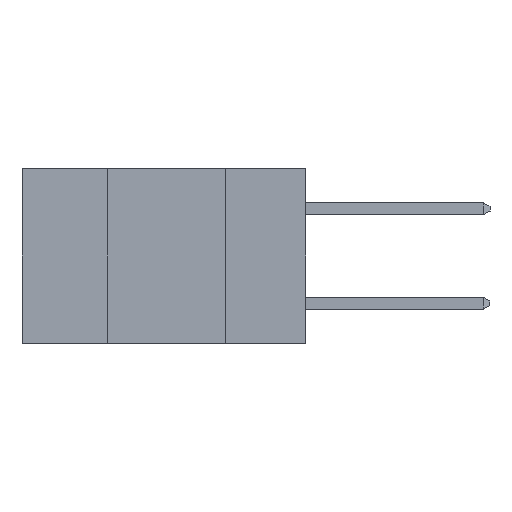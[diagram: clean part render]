
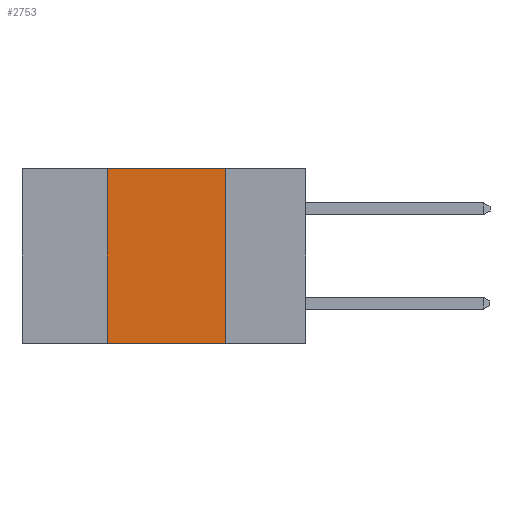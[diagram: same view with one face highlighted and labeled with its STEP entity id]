
A CAD part, left-side view. The second image highlights one B-rep face of the part: STEP entity #2753.
In plain terms, the highlighted planar face has unit normal (-1, 0, 0).
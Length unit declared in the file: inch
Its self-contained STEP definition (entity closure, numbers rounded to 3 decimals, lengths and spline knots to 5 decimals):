
#71 = VECTOR ( 'NONE', #6612, 39.37008 ) ;
#269 = VECTOR ( 'NONE', #9009, 39.37008 ) ;
#537 = CARTESIAN_POINT ( 'NONE',  ( 0., 0.6, -0.37 ) ) ;
#635 = VECTOR ( 'NONE', #5246, 39.37008 ) ;
#1013 = ORIENTED_EDGE ( 'NONE', *, *, #5475, .F. ) ;
#1156 = DIRECTION ( 'NONE',  ( 1., 0., 0. ) ) ;
#1180 = LINE ( 'NONE', #12051, #8700 ) ;
#1385 = PLANE ( 'NONE',  #6379 ) ;
#2689 = EDGE_LOOP ( 'NONE', ( #1013, #3523, #4507, #5567 ) ) ;
#2753 = ADVANCED_FACE ( 'NONE', ( #4590 ), #1385, .F. ) ;
#3091 = CARTESIAN_POINT ( 'NONE',  ( 0., 0.42, 0. ) ) ;
#3523 = ORIENTED_EDGE ( 'NONE', *, *, #11080, .F. ) ;
#3814 = DIRECTION ( 'NONE',  ( 0., 0., -1. ) ) ;
#4144 = VERTEX_POINT ( 'NONE', #3091 ) ;
#4183 = EDGE_CURVE ( 'NONE', #7644, #7170, #6390, .T. ) ;
#4507 = ORIENTED_EDGE ( 'NONE', *, *, #4842, .F. ) ;
#4590 = FACE_OUTER_BOUND ( 'NONE', #2689, .T. ) ;
#4842 = EDGE_CURVE ( 'NONE', #7644, #4144, #1180, .T. ) ;
#5246 = DIRECTION ( 'NONE',  ( 0., -1., 0. ) ) ;
#5475 = EDGE_CURVE ( 'NONE', #10749, #7170, #6062, .T. ) ;
#5567 = ORIENTED_EDGE ( 'NONE', *, *, #4183, .T. ) ;
#5872 = LINE ( 'NONE', #7511, #71 ) ;
#6062 = LINE ( 'NONE', #9321, #269 ) ;
#6379 = AXIS2_PLACEMENT_3D ( 'NONE', #6758, #1156, #3814 ) ;
#6390 = LINE ( 'NONE', #537, #635 ) ;
#6495 = CARTESIAN_POINT ( 'NONE',  ( 0., 0.17, -0.37 ) ) ;
#6612 = DIRECTION ( 'NONE',  ( 0., -1., 0. ) ) ;
#6758 = CARTESIAN_POINT ( 'NONE',  ( 0., 0.6, 0. ) ) ;
#7170 = VERTEX_POINT ( 'NONE', #6495 ) ;
#7511 = CARTESIAN_POINT ( 'NONE',  ( 0., 0.6, 0. ) ) ;
#7644 = VERTEX_POINT ( 'NONE', #8844 ) ;
#8700 = VECTOR ( 'NONE', #11730, 39.37008 ) ;
#8844 = CARTESIAN_POINT ( 'NONE',  ( 0., 0.42, -0.37 ) ) ;
#9009 = DIRECTION ( 'NONE',  ( 0., 0., -1. ) ) ;
#9321 = CARTESIAN_POINT ( 'NONE',  ( 0., 0.17, 0. ) ) ;
#10749 = VERTEX_POINT ( 'NONE', #12526 ) ;
#11080 = EDGE_CURVE ( 'NONE', #4144, #10749, #5872, .T. ) ;
#11730 = DIRECTION ( 'NONE',  ( 0., 0., 1. ) ) ;
#12051 = CARTESIAN_POINT ( 'NONE',  ( 0., 0.42, 0. ) ) ;
#12526 = CARTESIAN_POINT ( 'NONE',  ( 0., 0.17, 0. ) ) ;
